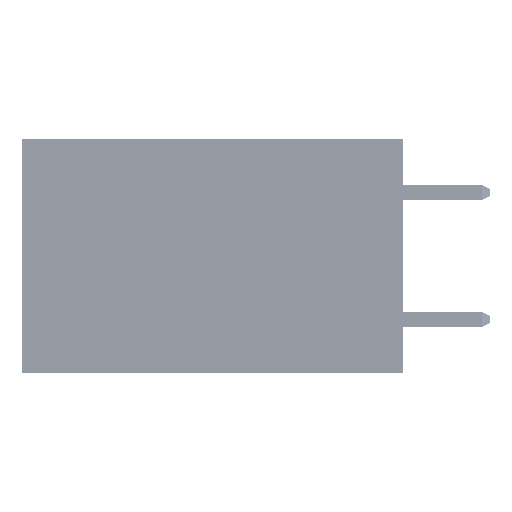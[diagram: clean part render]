
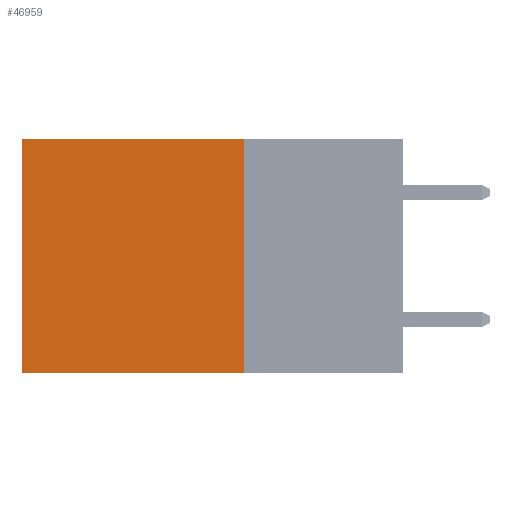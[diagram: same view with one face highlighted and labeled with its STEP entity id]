
A CAD part, left-side view. The second image highlights one B-rep face of the part: STEP entity #46959.
In plain terms, the highlighted planar face has unit normal (-1, 0, 0).
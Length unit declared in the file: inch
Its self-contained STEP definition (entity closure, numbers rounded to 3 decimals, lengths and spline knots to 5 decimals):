
#1956 = CARTESIAN_POINT ( 'NONE',  ( 0.2875, 0.25, 0. ) ) ;
#3005 = EDGE_CURVE ( 'NONE', #9022, #11557, #31699, .T. ) ;
#4059 = CARTESIAN_POINT ( 'NONE',  ( 0.2875, 0.6, 0. ) ) ;
#4400 = DIRECTION ( 'NONE',  ( 0., 0., -1. ) ) ;
#6434 = ORIENTED_EDGE ( 'NONE', *, *, #38292, .F. ) ;
#8584 = VECTOR ( 'NONE', #48697, 39.37008 ) ;
#8912 = VERTEX_POINT ( 'NONE', #18207 ) ;
#9022 = VERTEX_POINT ( 'NONE', #4059 ) ;
#9937 = AXIS2_PLACEMENT_3D ( 'NONE', #1956, #13239, #28293 ) ;
#10955 = LINE ( 'NONE', #17797, #13324 ) ;
#11557 = VERTEX_POINT ( 'NONE', #43095 ) ;
#13239 = DIRECTION ( 'NONE',  ( 1., 0., 0. ) ) ;
#13324 = VECTOR ( 'NONE', #32664, 39.37008 ) ;
#13401 = PLANE ( 'NONE',  #9937 ) ;
#17797 = CARTESIAN_POINT ( 'NONE',  ( 0.2875, 0.25, 0. ) ) ;
#18207 = CARTESIAN_POINT ( 'NONE',  ( 0.2875, 0.25, -0.37 ) ) ;
#20041 = CARTESIAN_POINT ( 'NONE',  ( 0.2875, 0.25, 0. ) ) ;
#21621 = VECTOR ( 'NONE', #4400, 39.37008 ) ;
#22162 = LINE ( 'NONE', #44864, #8584 ) ;
#23118 = CARTESIAN_POINT ( 'NONE',  ( 0.2875, 0.6, 0. ) ) ;
#23539 = LINE ( 'NONE', #38917, #30042 ) ;
#23776 = ORIENTED_EDGE ( 'NONE', *, *, #3005, .T. ) ;
#24900 = VERTEX_POINT ( 'NONE', #20041 ) ;
#28293 = DIRECTION ( 'NONE',  ( 0., 0., -1. ) ) ;
#30042 = VECTOR ( 'NONE', #38600, 39.37008 ) ;
#31699 = LINE ( 'NONE', #23118, #21621 ) ;
#32664 = DIRECTION ( 'NONE',  ( 0., 0., -1. ) ) ;
#33187 = EDGE_LOOP ( 'NONE', ( #23776, #6434, #40033, #36574 ) ) ;
#34662 = EDGE_CURVE ( 'NONE', #24900, #9022, #23539, .T. ) ;
#36574 = ORIENTED_EDGE ( 'NONE', *, *, #34662, .T. ) ;
#38292 = EDGE_CURVE ( 'NONE', #8912, #11557, #22162, .T. ) ;
#38600 = DIRECTION ( 'NONE',  ( 0., 1., 0. ) ) ;
#38917 = CARTESIAN_POINT ( 'NONE',  ( 0.2875, 0.25, 0. ) ) ;
#40033 = ORIENTED_EDGE ( 'NONE', *, *, #45801, .F. ) ;
#42172 = FACE_OUTER_BOUND ( 'NONE', #33187, .T. ) ;
#43095 = CARTESIAN_POINT ( 'NONE',  ( 0.2875, 0.6, -0.37 ) ) ;
#44864 = CARTESIAN_POINT ( 'NONE',  ( 0.2875, 0.25, -0.37 ) ) ;
#45801 = EDGE_CURVE ( 'NONE', #24900, #8912, #10955, .T. ) ;
#46959 = ADVANCED_FACE ( 'NONE', ( #42172 ), #13401, .F. ) ;
#48697 = DIRECTION ( 'NONE',  ( 0., 1., 0. ) ) ;
